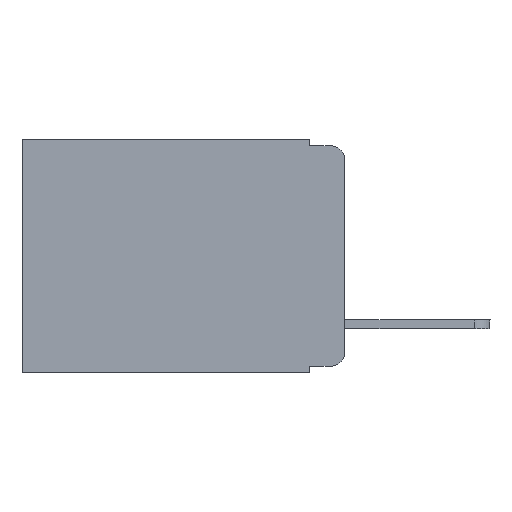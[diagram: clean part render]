
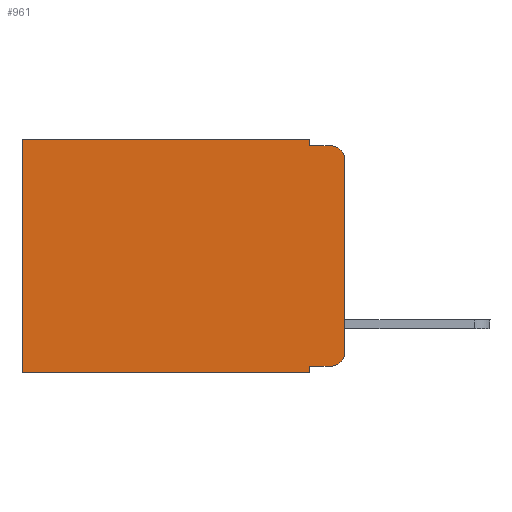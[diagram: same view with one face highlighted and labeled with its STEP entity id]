
A CAD part, left-side view. The second image highlights one B-rep face of the part: STEP entity #961.
In plain terms, the highlighted planar face has unit normal (-1, 0, 0).
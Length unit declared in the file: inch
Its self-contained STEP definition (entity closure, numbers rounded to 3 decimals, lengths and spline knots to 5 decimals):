
#601 = CIRCLE ( 'NONE', #11080, 0.02 ) ;
#645 = VERTEX_POINT ( 'NONE', #15516 ) ;
#961 = ADVANCED_FACE ( 'NONE', ( #20826 ), #9938, .F. ) ;
#1232 = DIRECTION ( 'NONE',  ( 0., 0., -1. ) ) ;
#1305 = EDGE_CURVE ( 'NONE', #5861, #16281, #5576, .T. ) ;
#1522 = EDGE_LOOP ( 'NONE', ( #6025, #5421, #18283, #18664, #5442, #15805, #6139, #7571, #7627, #2527 ) ) ;
#1983 = VERTEX_POINT ( 'NONE', #22079 ) ;
#2326 = EDGE_CURVE ( 'NONE', #645, #12744, #5785, .T. ) ;
#2527 = ORIENTED_EDGE ( 'NONE', *, *, #3580, .T. ) ;
#2541 = VECTOR ( 'NONE', #6378, 39.37008 ) ;
#3580 = EDGE_CURVE ( 'NONE', #9199, #21023, #601, .T. ) ;
#3980 = EDGE_CURVE ( 'NONE', #645, #13898, #13600, .T. ) ;
#4118 = DIRECTION ( 'NONE',  ( 0., 0., -1. ) ) ;
#4724 = DIRECTION ( 'NONE',  ( 0., -1., 0. ) ) ;
#5249 = VECTOR ( 'NONE', #19828, 39.37008 ) ;
#5301 = CARTESIAN_POINT ( 'NONE',  ( 0.298, 0., 0. ) ) ;
#5421 = ORIENTED_EDGE ( 'NONE', *, *, #6856, .T. ) ;
#5442 = ORIENTED_EDGE ( 'NONE', *, *, #2326, .T. ) ;
#5508 = EDGE_CURVE ( 'NONE', #13898, #1983, #11624, .T. ) ;
#5576 = LINE ( 'NONE', #18749, #19449 ) ;
#5785 = LINE ( 'NONE', #10935, #5249 ) ;
#5861 = VERTEX_POINT ( 'NONE', #19542 ) ;
#6025 = ORIENTED_EDGE ( 'NONE', *, *, #7225, .F. ) ;
#6139 = ORIENTED_EDGE ( 'NONE', *, *, #12476, .F. ) ;
#6378 = DIRECTION ( 'NONE',  ( 0., 1., 0. ) ) ;
#6641 = CARTESIAN_POINT ( 'NONE',  ( 0.298, 0.051, -0.01 ) ) ;
#6668 = DIRECTION ( 'NONE',  ( 0., 0., -1. ) ) ;
#6770 = LINE ( 'NONE', #5301, #7020 ) ;
#6793 = VECTOR ( 'NONE', #19048, 39.37008 ) ;
#6830 = CARTESIAN_POINT ( 'NONE',  ( 0.298, 0.051, -0.343 ) ) ;
#6856 = EDGE_CURVE ( 'NONE', #21522, #1983, #13580, .T. ) ;
#7020 = VECTOR ( 'NONE', #15571, 39.37008 ) ;
#7225 = EDGE_CURVE ( 'NONE', #21522, #21023, #6770, .T. ) ;
#7377 = AXIS2_PLACEMENT_3D ( 'NONE', #16794, #15101, #11694 ) ;
#7571 = ORIENTED_EDGE ( 'NONE', *, *, #1305, .F. ) ;
#7627 = ORIENTED_EDGE ( 'NONE', *, *, #16146, .T. ) ;
#7919 = CARTESIAN_POINT ( 'NONE',  ( 0.298, 0., -0.343 ) ) ;
#7951 = LINE ( 'NONE', #7919, #2541 ) ;
#8334 = DIRECTION ( 'NONE',  ( 0., 0., -1. ) ) ;
#8921 = CARTESIAN_POINT ( 'NONE',  ( 0.298, 0.02, -0.313 ) ) ;
#9199 = VERTEX_POINT ( 'NONE', #11503 ) ;
#9508 = CARTESIAN_POINT ( 'NONE',  ( 0.298, 0., -0.313 ) ) ;
#9816 = CARTESIAN_POINT ( 'NONE',  ( 0.298, 0.051, -0.333 ) ) ;
#9938 = PLANE ( 'NONE',  #7377 ) ;
#10935 = CARTESIAN_POINT ( 'NONE',  ( 0.298, 0., 0. ) ) ;
#11002 = DIRECTION ( 'NONE',  ( -1., 0., 0. ) ) ;
#11080 = AXIS2_PLACEMENT_3D ( 'NONE', #8921, #18090, #6668 ) ;
#11235 = CARTESIAN_POINT ( 'NONE',  ( 0.298, 0., -0.03 ) ) ;
#11503 = CARTESIAN_POINT ( 'NONE',  ( 0.298, 0.02, -0.333 ) ) ;
#11624 = LINE ( 'NONE', #18226, #13601 ) ;
#11694 = DIRECTION ( 'NONE',  ( 0., 0., -1. ) ) ;
#11879 = LINE ( 'NONE', #16714, #19223 ) ;
#12286 = AXIS2_PLACEMENT_3D ( 'NONE', #14488, #11002, #4118 ) ;
#12476 = EDGE_CURVE ( 'NONE', #16281, #15256, #7951, .T. ) ;
#12639 = CARTESIAN_POINT ( 'NONE',  ( 0.298, 0.473, -0.343 ) ) ;
#12744 = VERTEX_POINT ( 'NONE', #19075 ) ;
#12971 = VECTOR ( 'NONE', #4724, 39.37008 ) ;
#13580 = CIRCLE ( 'NONE', #12286, 0.02 ) ;
#13600 = LINE ( 'NONE', #22178, #6793 ) ;
#13601 = VECTOR ( 'NONE', #18374, 39.37008 ) ;
#13898 = VERTEX_POINT ( 'NONE', #6641 ) ;
#14488 = CARTESIAN_POINT ( 'NONE',  ( 0.298, 0.02, -0.03 ) ) ;
#15101 = DIRECTION ( 'NONE',  ( 1., 0., 0. ) ) ;
#15256 = VERTEX_POINT ( 'NONE', #12639 ) ;
#15516 = CARTESIAN_POINT ( 'NONE',  ( 0.298, 0.051, 0. ) ) ;
#15571 = DIRECTION ( 'NONE',  ( 0., 0., -1. ) ) ;
#15805 = ORIENTED_EDGE ( 'NONE', *, *, #19708, .T. ) ;
#16146 = EDGE_CURVE ( 'NONE', #5861, #9199, #16508, .T. ) ;
#16281 = VERTEX_POINT ( 'NONE', #6830 ) ;
#16508 = LINE ( 'NONE', #9816, #12971 ) ;
#16714 = CARTESIAN_POINT ( 'NONE',  ( 0.298, 0.473, 0. ) ) ;
#16794 = CARTESIAN_POINT ( 'NONE',  ( 0.298, 0., 0. ) ) ;
#18090 = DIRECTION ( 'NONE',  ( -1., 0., 0. ) ) ;
#18226 = CARTESIAN_POINT ( 'NONE',  ( 0.298, 0.051, -0.01 ) ) ;
#18283 = ORIENTED_EDGE ( 'NONE', *, *, #5508, .F. ) ;
#18374 = DIRECTION ( 'NONE',  ( 0., -1., 0. ) ) ;
#18664 = ORIENTED_EDGE ( 'NONE', *, *, #3980, .F. ) ;
#18749 = CARTESIAN_POINT ( 'NONE',  ( 0.298, 0.051, 0. ) ) ;
#19048 = DIRECTION ( 'NONE',  ( 0., 0., -1. ) ) ;
#19075 = CARTESIAN_POINT ( 'NONE',  ( 0.298, 0.473, 0. ) ) ;
#19223 = VECTOR ( 'NONE', #1232, 39.37008 ) ;
#19449 = VECTOR ( 'NONE', #8334, 39.37008 ) ;
#19542 = CARTESIAN_POINT ( 'NONE',  ( 0.298, 0.051, -0.333 ) ) ;
#19708 = EDGE_CURVE ( 'NONE', #12744, #15256, #11879, .T. ) ;
#19828 = DIRECTION ( 'NONE',  ( 0., 1., 0. ) ) ;
#20826 = FACE_OUTER_BOUND ( 'NONE', #1522, .T. ) ;
#21023 = VERTEX_POINT ( 'NONE', #9508 ) ;
#21522 = VERTEX_POINT ( 'NONE', #11235 ) ;
#22079 = CARTESIAN_POINT ( 'NONE',  ( 0.298, 0.02, -0.01 ) ) ;
#22178 = CARTESIAN_POINT ( 'NONE',  ( 0.298, 0.051, 0. ) ) ;
